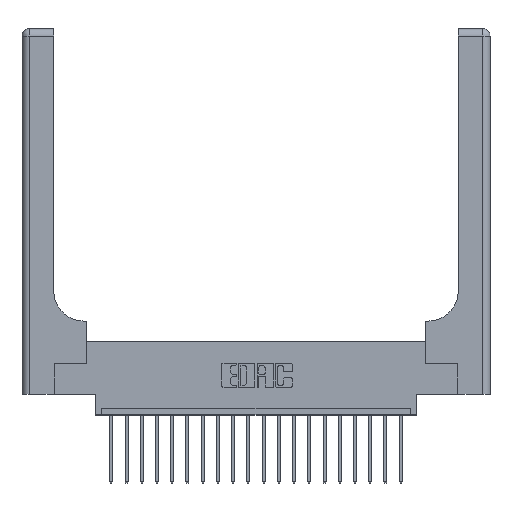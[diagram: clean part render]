
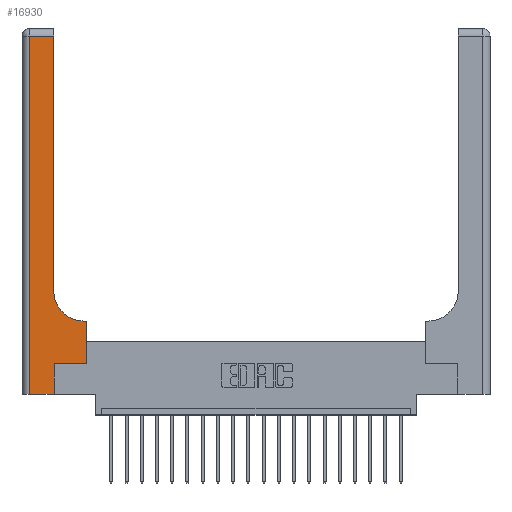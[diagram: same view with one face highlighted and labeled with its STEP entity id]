
A CAD part, top view. The second image highlights one B-rep face of the part: STEP entity #16930.
In plain terms, the highlighted planar face has unit normal (0, 0, 1).
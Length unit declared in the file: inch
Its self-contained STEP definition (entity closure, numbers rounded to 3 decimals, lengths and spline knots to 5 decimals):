
#505 = VECTOR ( 'NONE', #11041, 39.37008 ) ;
#917 = VECTOR ( 'NONE', #18141, 39.37008 ) ;
#941 = ORIENTED_EDGE ( 'NONE', *, *, #20004, .T. ) ;
#1439 = LINE ( 'NONE', #10471, #3961 ) ;
#1724 = DIRECTION ( 'NONE',  ( -1., 0., 0. ) ) ;
#1837 = CARTESIAN_POINT ( 'NONE',  ( 0.265, 0.25, 0.37 ) ) ;
#2199 = LINE ( 'NONE', #11259, #18740 ) ;
#2259 = VERTEX_POINT ( 'NONE', #6470 ) ;
#3222 = EDGE_CURVE ( 'NONE', #9050, #11813, #6820, .T. ) ;
#3350 = DIRECTION ( 'NONE',  ( 0., 0., -1. ) ) ;
#3440 = CARTESIAN_POINT ( 'NONE',  ( 0.26, 3., 0.37 ) ) ;
#3452 = CARTESIAN_POINT ( 'NONE',  ( 0.51, 0.6, 0.37 ) ) ;
#3554 = VERTEX_POINT ( 'NONE', #8729 ) ;
#3961 = VECTOR ( 'NONE', #9006, 39.37008 ) ;
#4305 = DIRECTION ( 'NONE',  ( -1., 0., 0. ) ) ;
#4414 = CARTESIAN_POINT ( 'NONE',  ( 0.265, 0., 0.37 ) ) ;
#4654 = DIRECTION ( 'NONE',  ( 0., 1., 0. ) ) ;
#5036 = EDGE_CURVE ( 'NONE', #12921, #20639, #16268, .T. ) ;
#5148 = ORIENTED_EDGE ( 'NONE', *, *, #14697, .T. ) ;
#5941 = LINE ( 'NONE', #1837, #10134 ) ;
#6173 = EDGE_CURVE ( 'NONE', #10580, #20488, #1439, .T. ) ;
#6470 = CARTESIAN_POINT ( 'NONE',  ( 0.06, 2.94, 0.37 ) ) ;
#6820 = LINE ( 'NONE', #14174, #14823 ) ;
#7963 = AXIS2_PLACEMENT_3D ( 'NONE', #20533, #15523, #4305 ) ;
#7972 = ORIENTED_EDGE ( 'NONE', *, *, #3222, .T. ) ;
#8205 = CARTESIAN_POINT ( 'NONE',  ( 0.26, 2.94, 0.37 ) ) ;
#8311 = VECTOR ( 'NONE', #9987, 39.37008 ) ;
#8467 = CARTESIAN_POINT ( 'NONE',  ( 0.265, 0.25, 0.37 ) ) ;
#8729 = CARTESIAN_POINT ( 'NONE',  ( 0.06, 0., 0.37 ) ) ;
#9006 = DIRECTION ( 'NONE',  ( 0., 1., 0. ) ) ;
#9050 = VERTEX_POINT ( 'NONE', #4414 ) ;
#9987 = DIRECTION ( 'NONE',  ( 0., -1., 0. ) ) ;
#10134 = VECTOR ( 'NONE', #15969, 39.37008 ) ;
#10340 = CARTESIAN_POINT ( 'NONE',  ( 0.26, 0.85, 0.37 ) ) ;
#10471 = CARTESIAN_POINT ( 'NONE',  ( 0.528, 0.25, 0.37 ) ) ;
#10580 = VERTEX_POINT ( 'NONE', #16029 ) ;
#10871 = ORIENTED_EDGE ( 'NONE', *, *, #13791, .T. ) ;
#11041 = DIRECTION ( 'NONE',  ( 1., 0., 0. ) ) ;
#11259 = CARTESIAN_POINT ( 'NONE',  ( 0.26, 0.6, 0.37 ) ) ;
#11332 = FACE_OUTER_BOUND ( 'NONE', #16542, .T. ) ;
#11519 = CARTESIAN_POINT ( 'NONE',  ( 0., 2.94, 0.37 ) ) ;
#11779 = LINE ( 'NONE', #14839, #8311 ) ;
#11813 = VERTEX_POINT ( 'NONE', #8467 ) ;
#12482 = VECTOR ( 'NONE', #14386, 39.37008 ) ;
#12921 = VERTEX_POINT ( 'NONE', #10340 ) ;
#13653 = LINE ( 'NONE', #11519, #917 ) ;
#13791 = EDGE_CURVE ( 'NONE', #20488, #18853, #2199, .T. ) ;
#13807 = EDGE_CURVE ( 'NONE', #18853, #12921, #14455, .T. ) ;
#14123 = PLANE ( 'NONE',  #7963 ) ;
#14174 = CARTESIAN_POINT ( 'NONE',  ( 0.265, 0., 0.37 ) ) ;
#14235 = ORIENTED_EDGE ( 'NONE', *, *, #14507, .T. ) ;
#14386 = DIRECTION ( 'NONE',  ( 0., 1., 0. ) ) ;
#14455 = CIRCLE ( 'NONE', #19824, 0.25 ) ;
#14501 = DIRECTION ( 'NONE',  ( 1., 0., 0. ) ) ;
#14507 = EDGE_CURVE ( 'NONE', #11813, #10580, #5941, .T. ) ;
#14697 = EDGE_CURVE ( 'NONE', #20639, #2259, #13653, .T. ) ;
#14823 = VECTOR ( 'NONE', #4654, 39.37008 ) ;
#14839 = CARTESIAN_POINT ( 'NONE',  ( 0.06, 3., 0.37 ) ) ;
#15523 = DIRECTION ( 'NONE',  ( 0., 0., -1. ) ) ;
#15756 = LINE ( 'NONE', #19062, #505 ) ;
#15969 = DIRECTION ( 'NONE',  ( 1., 0., 0. ) ) ;
#16029 = CARTESIAN_POINT ( 'NONE',  ( 0.528, 0.25, 0.37 ) ) ;
#16058 = ORIENTED_EDGE ( 'NONE', *, *, #5036, .T. ) ;
#16268 = LINE ( 'NONE', #3440, #12482 ) ;
#16542 = EDGE_LOOP ( 'NONE', ( #16058, #5148, #16674, #941, #7972, #14235, #16574, #10871, #19593 ) ) ;
#16574 = ORIENTED_EDGE ( 'NONE', *, *, #6173, .T. ) ;
#16674 = ORIENTED_EDGE ( 'NONE', *, *, #18368, .T. ) ;
#16930 = ADVANCED_FACE ( 'NONE', ( #11332 ), #14123, .F. ) ;
#17577 = CARTESIAN_POINT ( 'NONE',  ( 0.528, 0.6, 0.37 ) ) ;
#17684 = CARTESIAN_POINT ( 'NONE',  ( 0.51, 0.85, 0.37 ) ) ;
#18141 = DIRECTION ( 'NONE',  ( -1., 0., 0. ) ) ;
#18368 = EDGE_CURVE ( 'NONE', #2259, #3554, #11779, .T. ) ;
#18740 = VECTOR ( 'NONE', #1724, 39.37008 ) ;
#18853 = VERTEX_POINT ( 'NONE', #3452 ) ;
#19062 = CARTESIAN_POINT ( 'NONE',  ( 0., 0., 0.37 ) ) ;
#19593 = ORIENTED_EDGE ( 'NONE', *, *, #13807, .T. ) ;
#19824 = AXIS2_PLACEMENT_3D ( 'NONE', #17684, #3350, #14501 ) ;
#20004 = EDGE_CURVE ( 'NONE', #3554, #9050, #15756, .T. ) ;
#20488 = VERTEX_POINT ( 'NONE', #17577 ) ;
#20533 = CARTESIAN_POINT ( 'NONE',  ( 0., 3., 0.37 ) ) ;
#20639 = VERTEX_POINT ( 'NONE', #8205 ) ;
